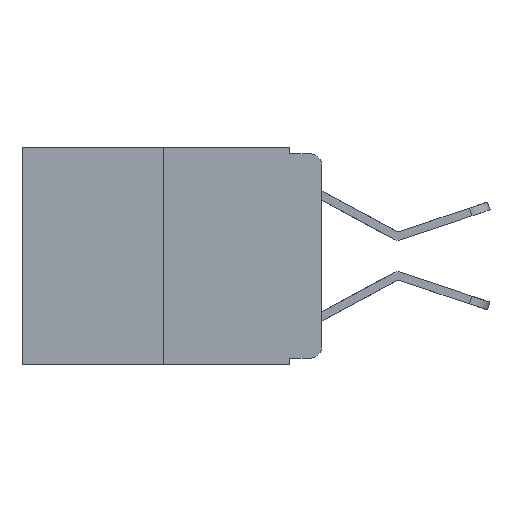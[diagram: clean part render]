
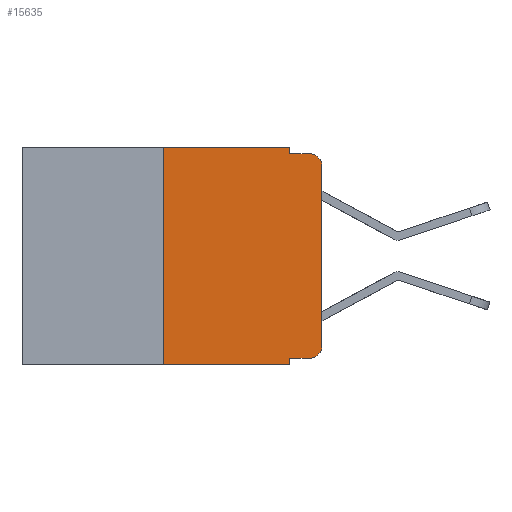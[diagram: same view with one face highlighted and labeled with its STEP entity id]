
A CAD part, left-side view. The second image highlights one B-rep face of the part: STEP entity #15635.
In plain terms, the highlighted planar face has unit normal (-1, 0, 0).
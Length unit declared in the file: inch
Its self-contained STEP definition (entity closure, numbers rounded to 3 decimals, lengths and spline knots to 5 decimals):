
#165 = CARTESIAN_POINT ( 'NONE',  ( 0., 0.051, -0.333 ) ) ;
#252 = PLANE ( 'NONE',  #2179 ) ;
#727 = VECTOR ( 'NONE', #2998, 39.37008 ) ;
#744 = CARTESIAN_POINT ( 'NONE',  ( 0., 0.25, 0. ) ) ;
#773 = EDGE_CURVE ( 'NONE', #5562, #15954, #6368, .T. ) ;
#1005 = EDGE_CURVE ( 'NONE', #18136, #1413, #17508, .T. ) ;
#1186 = ORIENTED_EDGE ( 'NONE', *, *, #9605, .F. ) ;
#1214 = VECTOR ( 'NONE', #16779, 39.37008 ) ;
#1329 = CARTESIAN_POINT ( 'NONE',  ( 0., 0.051, 0. ) ) ;
#1334 = DIRECTION ( 'NONE',  ( 0., -1., 0. ) ) ;
#1413 = VERTEX_POINT ( 'NONE', #19918 ) ;
#1670 = LINE ( 'NONE', #165, #727 ) ;
#2103 = LINE ( 'NONE', #3837, #18210 ) ;
#2142 = CARTESIAN_POINT ( 'NONE',  ( 0., 0.02, -0.03 ) ) ;
#2179 = AXIS2_PLACEMENT_3D ( 'NONE', #12655, #4981, #10869 ) ;
#2406 = CARTESIAN_POINT ( 'NONE',  ( 0., 0.051, 0. ) ) ;
#2511 = VECTOR ( 'NONE', #6669, 39.37008 ) ;
#2620 = DIRECTION ( 'NONE',  ( 0., -1., 0. ) ) ;
#2791 = AXIS2_PLACEMENT_3D ( 'NONE', #2142, #11450, #9933 ) ;
#2906 = ORIENTED_EDGE ( 'NONE', *, *, #16303, .F. ) ;
#2998 = DIRECTION ( 'NONE',  ( 0., -1., 0. ) ) ;
#3008 = ORIENTED_EDGE ( 'NONE', *, *, #9119, .T. ) ;
#3837 = CARTESIAN_POINT ( 'NONE',  ( 0., 0.051, 0. ) ) ;
#4171 = CARTESIAN_POINT ( 'NONE',  ( 0., 0.02, -0.333 ) ) ;
#4439 = ORIENTED_EDGE ( 'NONE', *, *, #17519, .T. ) ;
#4607 = ORIENTED_EDGE ( 'NONE', *, *, #14427, .T. ) ;
#4643 = ORIENTED_EDGE ( 'NONE', *, *, #1005, .F. ) ;
#4685 = FACE_OUTER_BOUND ( 'NONE', #14890, .T. ) ;
#4981 = DIRECTION ( 'NONE',  ( 1., 0., 0. ) ) ;
#5346 = EDGE_CURVE ( 'NONE', #19790, #5562, #1670, .T. ) ;
#5382 = ORIENTED_EDGE ( 'NONE', *, *, #5346, .T. ) ;
#5562 = VERTEX_POINT ( 'NONE', #4171 ) ;
#5810 = CARTESIAN_POINT ( 'NONE',  ( 0., 0.02, -0.313 ) ) ;
#5973 = CARTESIAN_POINT ( 'NONE',  ( 0., 0.02, -0.01 ) ) ;
#6368 = CIRCLE ( 'NONE', #13787, 0.02 ) ;
#6524 = VECTOR ( 'NONE', #11879, 39.37008 ) ;
#6669 = DIRECTION ( 'NONE',  ( 0., 0., 1. ) ) ;
#6943 = CARTESIAN_POINT ( 'NONE',  ( 0., 0.051, -0.343 ) ) ;
#7966 = CARTESIAN_POINT ( 'NONE',  ( 0., 0.051, -0.333 ) ) ;
#8342 = VECTOR ( 'NONE', #2620, 39.37008 ) ;
#8714 = CARTESIAN_POINT ( 'NONE',  ( 0., 0., -0.313 ) ) ;
#8926 = LINE ( 'NONE', #15076, #16869 ) ;
#9119 = EDGE_CURVE ( 'NONE', #18136, #19427, #13388, .T. ) ;
#9605 = EDGE_CURVE ( 'NONE', #14790, #17193, #8926, .T. ) ;
#9787 = CARTESIAN_POINT ( 'NONE',  ( 0., 0.25, -0.343 ) ) ;
#9879 = CARTESIAN_POINT ( 'NONE',  ( 0., 0.051, -0.01 ) ) ;
#9933 = DIRECTION ( 'NONE',  ( 0., 0., -1. ) ) ;
#10869 = DIRECTION ( 'NONE',  ( 0., 0., -1. ) ) ;
#10944 = ORIENTED_EDGE ( 'NONE', *, *, #19366, .F. ) ;
#11273 = DIRECTION ( 'NONE',  ( 0., 0., 1. ) ) ;
#11450 = DIRECTION ( 'NONE',  ( -1., 0., 0. ) ) ;
#11879 = DIRECTION ( 'NONE',  ( 0., -1., 0. ) ) ;
#12088 = VERTEX_POINT ( 'NONE', #2406 ) ;
#12405 = ORIENTED_EDGE ( 'NONE', *, *, #17198, .F. ) ;
#12655 = CARTESIAN_POINT ( 'NONE',  ( 0., 0.473, 0. ) ) ;
#12918 = DIRECTION ( 'NONE',  ( 0., 0., -1. ) ) ;
#13142 = CARTESIAN_POINT ( 'NONE',  ( 0., 0., 0. ) ) ;
#13388 = LINE ( 'NONE', #19539, #6524 ) ;
#13787 = AXIS2_PLACEMENT_3D ( 'NONE', #5810, #15004, #19444 ) ;
#14427 = EDGE_CURVE ( 'NONE', #18729, #17193, #15056, .T. ) ;
#14550 = LINE ( 'NONE', #13142, #2511 ) ;
#14790 = VERTEX_POINT ( 'NONE', #9879 ) ;
#14890 = EDGE_LOOP ( 'NONE', ( #4439, #4607, #1186, #10944, #2906, #4643, #3008, #12405, #5382, #18821 ) ) ;
#15004 = DIRECTION ( 'NONE',  ( -1., 0., 0. ) ) ;
#15044 = CARTESIAN_POINT ( 'NONE',  ( 0., 0.473, 0. ) ) ;
#15056 = CIRCLE ( 'NONE', #2791, 0.02 ) ;
#15076 = CARTESIAN_POINT ( 'NONE',  ( 0., 0.051, -0.01 ) ) ;
#15635 = ADVANCED_FACE ( 'NONE', ( #4685 ), #252, .F. ) ;
#15954 = VERTEX_POINT ( 'NONE', #8714 ) ;
#16303 = EDGE_CURVE ( 'NONE', #1413, #12088, #17864, .T. ) ;
#16779 = DIRECTION ( 'NONE',  ( 0., 0., -1. ) ) ;
#16869 = VECTOR ( 'NONE', #1334, 39.37008 ) ;
#17193 = VERTEX_POINT ( 'NONE', #5973 ) ;
#17198 = EDGE_CURVE ( 'NONE', #19790, #19427, #18094, .T. ) ;
#17282 = CARTESIAN_POINT ( 'NONE',  ( 0., 0., -0.03 ) ) ;
#17508 = LINE ( 'NONE', #744, #19603 ) ;
#17519 = EDGE_CURVE ( 'NONE', #15954, #18729, #14550, .T. ) ;
#17864 = LINE ( 'NONE', #15044, #8342 ) ;
#18094 = LINE ( 'NONE', #1329, #1214 ) ;
#18136 = VERTEX_POINT ( 'NONE', #9787 ) ;
#18210 = VECTOR ( 'NONE', #12918, 39.37008 ) ;
#18729 = VERTEX_POINT ( 'NONE', #17282 ) ;
#18821 = ORIENTED_EDGE ( 'NONE', *, *, #773, .T. ) ;
#19366 = EDGE_CURVE ( 'NONE', #12088, #14790, #2103, .T. ) ;
#19427 = VERTEX_POINT ( 'NONE', #6943 ) ;
#19444 = DIRECTION ( 'NONE',  ( 0., 0., -1. ) ) ;
#19539 = CARTESIAN_POINT ( 'NONE',  ( 0., 0.473, -0.343 ) ) ;
#19603 = VECTOR ( 'NONE', #11273, 39.37008 ) ;
#19790 = VERTEX_POINT ( 'NONE', #7966 ) ;
#19918 = CARTESIAN_POINT ( 'NONE',  ( 0., 0.25, 0. ) ) ;
